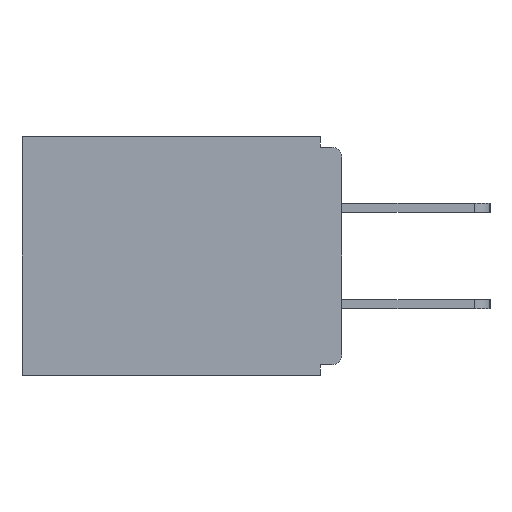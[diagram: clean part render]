
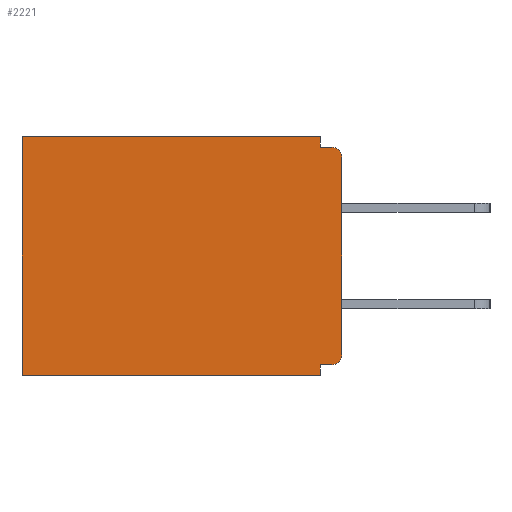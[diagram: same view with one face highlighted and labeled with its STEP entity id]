
A CAD part, left-side view. The second image highlights one B-rep face of the part: STEP entity #2221.
In plain terms, the highlighted planar face has unit normal (-1, 0, 0).
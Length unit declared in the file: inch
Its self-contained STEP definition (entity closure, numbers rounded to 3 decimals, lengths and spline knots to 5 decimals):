
#95 = EDGE_CURVE ( 'NONE', #9810, #10763, #6691, .T. ) ;
#368 = CARTESIAN_POINT ( 'NONE',  ( 0.298, 0., -0.328 ) ) ;
#528 = VECTOR ( 'NONE', #13909, 39.37008 ) ;
#618 = VERTEX_POINT ( 'NONE', #9127 ) ;
#735 = DIRECTION ( 'NONE',  ( 1., 0., 0. ) ) ;
#859 = VECTOR ( 'NONE', #2726, 39.37008 ) ;
#864 = ORIENTED_EDGE ( 'NONE', *, *, #7422, .F. ) ;
#1211 = EDGE_CURVE ( 'NONE', #7564, #10907, #6216, .T. ) ;
#1279 = DIRECTION ( 'NONE',  ( 0., 0., -1. ) ) ;
#1472 = EDGE_CURVE ( 'NONE', #1611, #9810, #7966, .T. ) ;
#1611 = VERTEX_POINT ( 'NONE', #4434 ) ;
#1817 = CARTESIAN_POINT ( 'NONE',  ( 0.298, 0., -0.03 ) ) ;
#1851 = CARTESIAN_POINT ( 'NONE',  ( 0.298, 0.015, -0.015 ) ) ;
#1960 = ORIENTED_EDGE ( 'NONE', *, *, #9380, .T. ) ;
#2221 = ADVANCED_FACE ( 'NONE', ( #3931 ), #13982, .F. ) ;
#2726 = DIRECTION ( 'NONE',  ( 0., 1., 0. ) ) ;
#3397 = ORIENTED_EDGE ( 'NONE', *, *, #95, .T. ) ;
#3504 = AXIS2_PLACEMENT_3D ( 'NONE', #13668, #12660, #10432 ) ;
#3551 = EDGE_CURVE ( 'NONE', #1611, #7564, #7560, .T. ) ;
#3931 = FACE_OUTER_BOUND ( 'NONE', #8367, .T. ) ;
#3949 = VECTOR ( 'NONE', #8838, 39.37008 ) ;
#4419 = AXIS2_PLACEMENT_3D ( 'NONE', #5090, #735, #8626 ) ;
#4434 = CARTESIAN_POINT ( 'NONE',  ( 0.298, 0.031, 0. ) ) ;
#4784 = CARTESIAN_POINT ( 'NONE',  ( 0.298, 0.031, -0.343 ) ) ;
#5090 = CARTESIAN_POINT ( 'NONE',  ( 0.298, 0., 0. ) ) ;
#5192 = DIRECTION ( 'NONE',  ( 0., 1., 0. ) ) ;
#5203 = DIRECTION ( 'NONE',  ( 0., -1., 0. ) ) ;
#5279 = CARTESIAN_POINT ( 'NONE',  ( 0.298, 0., 0. ) ) ;
#5283 = LINE ( 'NONE', #4784, #11548 ) ;
#5399 = DIRECTION ( 'NONE',  ( -1., 0., 0. ) ) ;
#5423 = CARTESIAN_POINT ( 'NONE',  ( 0.298, 0.031, -0.328 ) ) ;
#5427 = CARTESIAN_POINT ( 'NONE',  ( 0.298, 0.031, -0.343 ) ) ;
#5526 = VECTOR ( 'NONE', #5192, 39.37008 ) ;
#5561 = ORIENTED_EDGE ( 'NONE', *, *, #14106, .F. ) ;
#6105 = ORIENTED_EDGE ( 'NONE', *, *, #13835, .F. ) ;
#6216 = LINE ( 'NONE', #12641, #13860 ) ;
#6691 = LINE ( 'NONE', #12857, #528 ) ;
#6815 = CARTESIAN_POINT ( 'NONE',  ( 0.298, 0.46, 0. ) ) ;
#6829 = ORIENTED_EDGE ( 'NONE', *, *, #1211, .F. ) ;
#6889 = LINE ( 'NONE', #368, #3949 ) ;
#7143 = CARTESIAN_POINT ( 'NONE',  ( 0.298, 0., -0.343 ) ) ;
#7422 = EDGE_CURVE ( 'NONE', #618, #10763, #7745, .T. ) ;
#7560 = LINE ( 'NONE', #5427, #7896 ) ;
#7564 = VERTEX_POINT ( 'NONE', #12816 ) ;
#7745 = LINE ( 'NONE', #7143, #859 ) ;
#7896 = VECTOR ( 'NONE', #1279, 39.37008 ) ;
#7900 = CARTESIAN_POINT ( 'NONE',  ( 0.298, 0., -0.313 ) ) ;
#7966 = LINE ( 'NONE', #5279, #5526 ) ;
#7969 = CIRCLE ( 'NONE', #8804, 0.015 ) ;
#8117 = ORIENTED_EDGE ( 'NONE', *, *, #1472, .T. ) ;
#8367 = EDGE_LOOP ( 'NONE', ( #14191, #6829, #10712, #8117, #3397, #864, #5561, #10724, #1960, #6105 ) ) ;
#8424 = CARTESIAN_POINT ( 'NONE',  ( 0.298, 0., 0. ) ) ;
#8529 = DIRECTION ( 'NONE',  ( 0., 0., -1. ) ) ;
#8626 = DIRECTION ( 'NONE',  ( 0., 0., -1. ) ) ;
#8804 = AXIS2_PLACEMENT_3D ( 'NONE', #9755, #5399, #13229 ) ;
#8838 = DIRECTION ( 'NONE',  ( 0., 1., 0. ) ) ;
#9127 = CARTESIAN_POINT ( 'NONE',  ( 0.298, 0.031, -0.343 ) ) ;
#9298 = VERTEX_POINT ( 'NONE', #5423 ) ;
#9380 = EDGE_CURVE ( 'NONE', #13589, #10438, #13567, .T. ) ;
#9755 = CARTESIAN_POINT ( 'NONE',  ( 0.298, 0.015, -0.03 ) ) ;
#9810 = VERTEX_POINT ( 'NONE', #6815 ) ;
#10432 = DIRECTION ( 'NONE',  ( 0., 0., -1. ) ) ;
#10438 = VERTEX_POINT ( 'NONE', #7900 ) ;
#10712 = ORIENTED_EDGE ( 'NONE', *, *, #3551, .F. ) ;
#10724 = ORIENTED_EDGE ( 'NONE', *, *, #11637, .F. ) ;
#10763 = VERTEX_POINT ( 'NONE', #11511 ) ;
#10907 = VERTEX_POINT ( 'NONE', #1851 ) ;
#11285 = CARTESIAN_POINT ( 'NONE',  ( 0.298, 0.015, -0.328 ) ) ;
#11492 = EDGE_CURVE ( 'NONE', #13819, #10907, #7969, .T. ) ;
#11511 = CARTESIAN_POINT ( 'NONE',  ( 0.298, 0.46, -0.343 ) ) ;
#11548 = VECTOR ( 'NONE', #12626, 39.37008 ) ;
#11637 = EDGE_CURVE ( 'NONE', #13589, #9298, #6889, .T. ) ;
#12434 = VECTOR ( 'NONE', #8529, 39.37008 ) ;
#12626 = DIRECTION ( 'NONE',  ( 0., 0., -1. ) ) ;
#12641 = CARTESIAN_POINT ( 'NONE',  ( 0.298, 0., -0.015 ) ) ;
#12660 = DIRECTION ( 'NONE',  ( -1., 0., 0. ) ) ;
#12816 = CARTESIAN_POINT ( 'NONE',  ( 0.298, 0.031, -0.015 ) ) ;
#12857 = CARTESIAN_POINT ( 'NONE',  ( 0.298, 0.46, 0. ) ) ;
#13229 = DIRECTION ( 'NONE',  ( 0., 0., -1. ) ) ;
#13460 = LINE ( 'NONE', #8424, #12434 ) ;
#13567 = CIRCLE ( 'NONE', #3504, 0.015 ) ;
#13589 = VERTEX_POINT ( 'NONE', #11285 ) ;
#13668 = CARTESIAN_POINT ( 'NONE',  ( 0.298, 0.015, -0.313 ) ) ;
#13819 = VERTEX_POINT ( 'NONE', #1817 ) ;
#13835 = EDGE_CURVE ( 'NONE', #13819, #10438, #13460, .T. ) ;
#13860 = VECTOR ( 'NONE', #5203, 39.37008 ) ;
#13909 = DIRECTION ( 'NONE',  ( 0., 0., -1. ) ) ;
#13982 = PLANE ( 'NONE',  #4419 ) ;
#14106 = EDGE_CURVE ( 'NONE', #9298, #618, #5283, .T. ) ;
#14191 = ORIENTED_EDGE ( 'NONE', *, *, #11492, .T. ) ;
